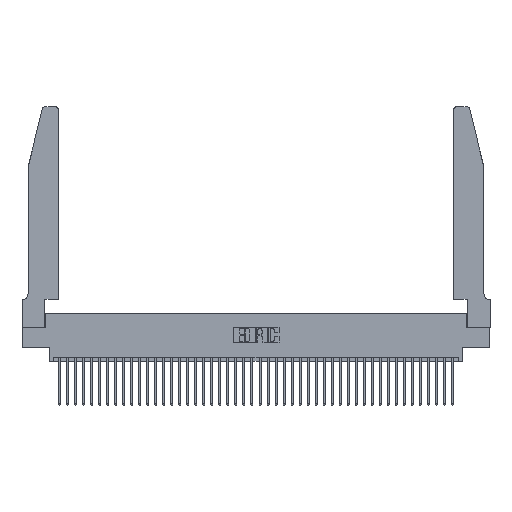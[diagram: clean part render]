
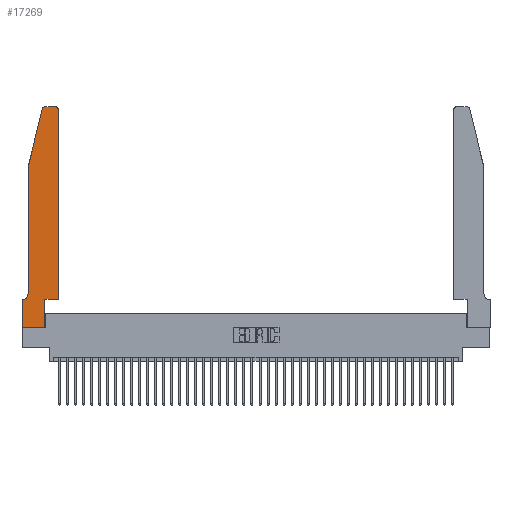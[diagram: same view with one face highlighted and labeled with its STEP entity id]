
A CAD part, top view. The second image highlights one B-rep face of the part: STEP entity #17269.
In plain terms, the highlighted planar face has unit normal (0, 0, 1).
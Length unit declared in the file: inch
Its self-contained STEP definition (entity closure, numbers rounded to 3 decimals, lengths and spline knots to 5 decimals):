
#984 = CARTESIAN_POINT ( 'NONE',  ( 0.284, 2.75, 0.37 ) ) ;
#1618 = CARTESIAN_POINT ( 'NONE',  ( 0.2605, 2.75, 0.37 ) ) ;
#1689 = CARTESIAN_POINT ( 'NONE',  ( 0.0055, 0.35, 0.37 ) ) ;
#4022 = LINE ( 'NONE', #37111, #18613 ) ;
#4811 = CARTESIAN_POINT ( 'NONE',  ( 0.4205, 2.75, 0.37 ) ) ;
#5225 = DIRECTION ( 'NONE',  ( 0., 0., -1. ) ) ;
#5644 = LINE ( 'NONE', #26296, #22290 ) ;
#6698 = CIRCLE ( 'NONE', #21180, 0.07 ) ;
#6991 = CARTESIAN_POINT ( 'NONE',  ( 0.4505, 0.35, 0.37 ) ) ;
#7086 = ORIENTED_EDGE ( 'NONE', *, *, #12168, .T. ) ;
#7139 = AXIS2_PLACEMENT_3D ( 'NONE', #11422, #30883, #17614 ) ;
#7619 = VECTOR ( 'NONE', #23605, 39.37008 ) ;
#8762 = CARTESIAN_POINT ( 'NONE',  ( 0., 0.35, 0.37 ) ) ;
#10048 = VERTEX_POINT ( 'NONE', #33732 ) ;
#10248 = ORIENTED_EDGE ( 'NONE', *, *, #14375, .T. ) ;
#10292 = ORIENTED_EDGE ( 'NONE', *, *, #40144, .T. ) ;
#10540 = EDGE_CURVE ( 'NONE', #26379, #11066, #31339, .T. ) ;
#10894 = AXIS2_PLACEMENT_3D ( 'NONE', #38091, #34788, #21197 ) ;
#10927 = ORIENTED_EDGE ( 'NONE', *, *, #38557, .T. ) ;
#11048 = VECTOR ( 'NONE', #19149, 39.37008 ) ;
#11054 = LINE ( 'NONE', #12320, #33923 ) ;
#11066 = VERTEX_POINT ( 'NONE', #36131 ) ;
#11199 = DIRECTION ( 'NONE',  ( 0., -1., 0. ) ) ;
#11422 = CARTESIAN_POINT ( 'NONE',  ( 0., 0.35, 0.37 ) ) ;
#11558 = PLANE ( 'NONE',  #7139 ) ;
#12168 = EDGE_CURVE ( 'NONE', #10048, #15515, #6698, .T. ) ;
#12319 = LINE ( 'NONE', #20229, #42028 ) ;
#12320 = CARTESIAN_POINT ( 'NONE',  ( 0.0755, 0.35, 0.37 ) ) ;
#12638 = DIRECTION ( 'NONE',  ( 0., 1., 0. ) ) ;
#13358 = EDGE_CURVE ( 'NONE', #22673, #25272, #32654, .T. ) ;
#14375 = EDGE_CURVE ( 'NONE', #16214, #22673, #40339, .T. ) ;
#14385 = CIRCLE ( 'NONE', #10894, 0.03 ) ;
#14867 = CARTESIAN_POINT ( 'NONE',  ( 0.2865, 0.35, 0.37 ) ) ;
#15515 = VERTEX_POINT ( 'NONE', #1689 ) ;
#16214 = VERTEX_POINT ( 'NONE', #18883 ) ;
#17205 = CARTESIAN_POINT ( 'NONE',  ( 0.2865, 0.35, 0.37 ) ) ;
#17269 = ADVANCED_FACE ( 'NONE', ( #27584 ), #11558, .T. ) ;
#17614 = DIRECTION ( 'NONE',  ( 1., 0., 0. ) ) ;
#18613 = VECTOR ( 'NONE', #40464, 39.37008 ) ;
#18654 = EDGE_CURVE ( 'NONE', #36128, #16214, #5644, .T. ) ;
#18883 = CARTESIAN_POINT ( 'NONE',  ( 0.4505, 2.72, 0.37 ) ) ;
#19116 = LINE ( 'NONE', #20284, #7619 ) ;
#19149 = DIRECTION ( 'NONE',  ( 0., -1., 0. ) ) ;
#19261 = ORIENTED_EDGE ( 'NONE', *, *, #26099, .T. ) ;
#19592 = ORIENTED_EDGE ( 'NONE', *, *, #39068, .T. ) ;
#19780 = CARTESIAN_POINT ( 'NONE',  ( 0.0755, 2., 0.37 ) ) ;
#19878 = CARTESIAN_POINT ( 'NONE',  ( 0.4205, 2.72, 0.37 ) ) ;
#20012 = DIRECTION ( 'NONE',  ( 0., 1., 0. ) ) ;
#20229 = CARTESIAN_POINT ( 'NONE',  ( 0.4505, 0.35, 0.37 ) ) ;
#20284 = CARTESIAN_POINT ( 'NONE',  ( 0.0755, 2., 0.37 ) ) ;
#20315 = DIRECTION ( 'NONE',  ( 0., 0., 1. ) ) ;
#20456 = AXIS2_PLACEMENT_3D ( 'NONE', #19878, #20315, #25995 ) ;
#20731 = CARTESIAN_POINT ( 'NONE',  ( 0.0055, 0.42, 0.37 ) ) ;
#21180 = AXIS2_PLACEMENT_3D ( 'NONE', #20731, #5225, #22088 ) ;
#21197 = DIRECTION ( 'NONE',  ( 1., 0., 0. ) ) ;
#21243 = LINE ( 'NONE', #30530, #28054 ) ;
#22088 = DIRECTION ( 'NONE',  ( -1., 0., 0. ) ) ;
#22290 = VECTOR ( 'NONE', #12638, 39.37008 ) ;
#22673 = VERTEX_POINT ( 'NONE', #4811 ) ;
#23037 = EDGE_CURVE ( 'NONE', #15515, #26379, #11054, .T. ) ;
#23605 = DIRECTION ( 'NONE',  ( -0.239, -0.971, 0. ) ) ;
#24563 = DIRECTION ( 'NONE',  ( -1., 0., 0. ) ) ;
#24564 = ORIENTED_EDGE ( 'NONE', *, *, #10540, .T. ) ;
#24825 = VECTOR ( 'NONE', #24563, 39.37008 ) ;
#25272 = VERTEX_POINT ( 'NONE', #984 ) ;
#25995 = DIRECTION ( 'NONE',  ( 1., 0., 0. ) ) ;
#26055 = ORIENTED_EDGE ( 'NONE', *, *, #23037, .T. ) ;
#26099 = EDGE_CURVE ( 'NONE', #33511, #31428, #19116, .T. ) ;
#26296 = CARTESIAN_POINT ( 'NONE',  ( 0.4505, 0.35, 0.37 ) ) ;
#26379 = VERTEX_POINT ( 'NONE', #8762 ) ;
#27584 = FACE_OUTER_BOUND ( 'NONE', #28362, .T. ) ;
#27915 = VERTEX_POINT ( 'NONE', #14867 ) ;
#28054 = VECTOR ( 'NONE', #11199, 39.37008 ) ;
#28362 = EDGE_LOOP ( 'NONE', ( #37110, #36185, #19261, #10927, #7086, #26055, #24564, #10292, #19592, #41708, #30463, #10248 ) ) ;
#28798 = DIRECTION ( 'NONE',  ( -1., 0., 0. ) ) ;
#30287 = DIRECTION ( 'NONE',  ( 1., 0., 0. ) ) ;
#30463 = ORIENTED_EDGE ( 'NONE', *, *, #18654, .T. ) ;
#30530 = CARTESIAN_POINT ( 'NONE',  ( 0.0755, 2., 0.37 ) ) ;
#30883 = DIRECTION ( 'NONE',  ( 0., 0., 1. ) ) ;
#31339 = LINE ( 'NONE', #39404, #11048 ) ;
#31428 = VERTEX_POINT ( 'NONE', #19780 ) ;
#32654 = LINE ( 'NONE', #1618, #24825 ) ;
#32806 = VERTEX_POINT ( 'NONE', #41395 ) ;
#33342 = EDGE_CURVE ( 'NONE', #27915, #36128, #12319, .T. ) ;
#33511 = VERTEX_POINT ( 'NONE', #41045 ) ;
#33732 = CARTESIAN_POINT ( 'NONE',  ( 0.0755, 0.42, 0.37 ) ) ;
#33923 = VECTOR ( 'NONE', #28798, 39.37008 ) ;
#34082 = EDGE_CURVE ( 'NONE', #25272, #33511, #14385, .T. ) ;
#34788 = DIRECTION ( 'NONE',  ( 0., 0., 1. ) ) ;
#36128 = VERTEX_POINT ( 'NONE', #6991 ) ;
#36131 = CARTESIAN_POINT ( 'NONE',  ( 0., 0., 0.37 ) ) ;
#36185 = ORIENTED_EDGE ( 'NONE', *, *, #34082, .T. ) ;
#36835 = LINE ( 'NONE', #17205, #41541 ) ;
#37110 = ORIENTED_EDGE ( 'NONE', *, *, #13358, .T. ) ;
#37111 = CARTESIAN_POINT ( 'NONE',  ( 0., 0., 0.37 ) ) ;
#38091 = CARTESIAN_POINT ( 'NONE',  ( 0.284, 2.72, 0.37 ) ) ;
#38557 = EDGE_CURVE ( 'NONE', #31428, #10048, #21243, .T. ) ;
#39068 = EDGE_CURVE ( 'NONE', #32806, #27915, #36835, .T. ) ;
#39404 = CARTESIAN_POINT ( 'NONE',  ( 0., 0., 0.37 ) ) ;
#40144 = EDGE_CURVE ( 'NONE', #11066, #32806, #4022, .T. ) ;
#40339 = CIRCLE ( 'NONE', #20456, 0.03 ) ;
#40464 = DIRECTION ( 'NONE',  ( 1., 0., 0. ) ) ;
#41045 = CARTESIAN_POINT ( 'NONE',  ( 0.25487, 2.72718, 0.37 ) ) ;
#41395 = CARTESIAN_POINT ( 'NONE',  ( 0.2865, 0., 0.37 ) ) ;
#41541 = VECTOR ( 'NONE', #20012, 39.37008 ) ;
#41708 = ORIENTED_EDGE ( 'NONE', *, *, #33342, .T. ) ;
#42028 = VECTOR ( 'NONE', #30287, 39.37008 ) ;
